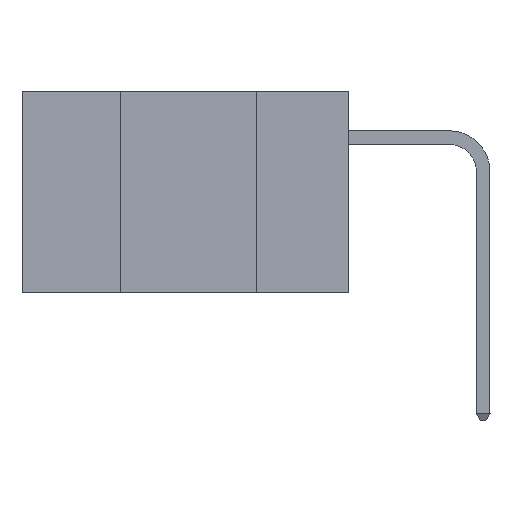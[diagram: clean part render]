
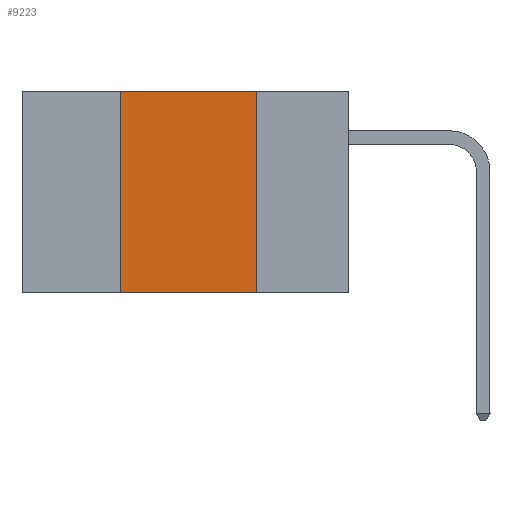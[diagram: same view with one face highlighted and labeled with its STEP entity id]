
A CAD part, left-side view. The second image highlights one B-rep face of the part: STEP entity #9223.
In plain terms, the highlighted planar face has unit normal (-1, 0, 0).
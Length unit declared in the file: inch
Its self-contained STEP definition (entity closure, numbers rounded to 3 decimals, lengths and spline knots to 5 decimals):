
#1359 = FACE_OUTER_BOUND ( 'NONE', #4938, .T. ) ;
#1415 = ORIENTED_EDGE ( 'NONE', *, *, #11528, .T. ) ;
#1892 = CARTESIAN_POINT ( 'NONE',  ( 0., 0.42, 0. ) ) ;
#2426 = VERTEX_POINT ( 'NONE', #2883 ) ;
#2479 = VERTEX_POINT ( 'NONE', #22346 ) ;
#2518 = LINE ( 'NONE', #7967, #10615 ) ;
#2652 = VERTEX_POINT ( 'NONE', #18044 ) ;
#2674 = VECTOR ( 'NONE', #9977, 39.37008 ) ;
#2860 = DIRECTION ( 'NONE',  ( 0., -1., 0. ) ) ;
#2883 = CARTESIAN_POINT ( 'NONE',  ( 0., 0.17, 0. ) ) ;
#3925 = DIRECTION ( 'NONE',  ( 0., 0., 1. ) ) ;
#4135 = ORIENTED_EDGE ( 'NONE', *, *, #16929, .F. ) ;
#4603 = DIRECTION ( 'NONE',  ( 0., -1., 0. ) ) ;
#4938 = EDGE_LOOP ( 'NONE', ( #17489, #9684, #4135, #1415 ) ) ;
#6083 = LINE ( 'NONE', #22148, #12660 ) ;
#6892 = CARTESIAN_POINT ( 'NONE',  ( 0., 0.17, 0. ) ) ;
#7019 = EDGE_CURVE ( 'NONE', #2652, #2426, #2518, .T. ) ;
#7704 = VECTOR ( 'NONE', #3925, 39.37008 ) ;
#7967 = CARTESIAN_POINT ( 'NONE',  ( 0., 0.6, 0. ) ) ;
#9223 = ADVANCED_FACE ( 'NONE', ( #1359 ), #18682, .F. ) ;
#9229 = EDGE_CURVE ( 'NONE', #2426, #10428, #13703, .T. ) ;
#9684 = ORIENTED_EDGE ( 'NONE', *, *, #7019, .F. ) ;
#9977 = DIRECTION ( 'NONE',  ( 0., 0., -1. ) ) ;
#10191 = DIRECTION ( 'NONE',  ( 1., 0., 0. ) ) ;
#10428 = VERTEX_POINT ( 'NONE', #20790 ) ;
#10615 = VECTOR ( 'NONE', #2860, 39.37008 ) ;
#11528 = EDGE_CURVE ( 'NONE', #2479, #10428, #6083, .T. ) ;
#12660 = VECTOR ( 'NONE', #4603, 39.37008 ) ;
#13703 = LINE ( 'NONE', #6892, #2674 ) ;
#15738 = LINE ( 'NONE', #1892, #7704 ) ;
#16929 = EDGE_CURVE ( 'NONE', #2479, #2652, #15738, .T. ) ;
#17489 = ORIENTED_EDGE ( 'NONE', *, *, #9229, .F. ) ;
#18044 = CARTESIAN_POINT ( 'NONE',  ( 0., 0.42, 0. ) ) ;
#18682 = PLANE ( 'NONE',  #21118 ) ;
#20252 = DIRECTION ( 'NONE',  ( 0., 0., -1. ) ) ;
#20485 = CARTESIAN_POINT ( 'NONE',  ( 0., 0.6, 0. ) ) ;
#20790 = CARTESIAN_POINT ( 'NONE',  ( 0., 0.17, -0.37 ) ) ;
#21118 = AXIS2_PLACEMENT_3D ( 'NONE', #20485, #10191, #20252 ) ;
#22148 = CARTESIAN_POINT ( 'NONE',  ( 0., 0.6, -0.37 ) ) ;
#22346 = CARTESIAN_POINT ( 'NONE',  ( 0., 0.42, -0.37 ) ) ;
